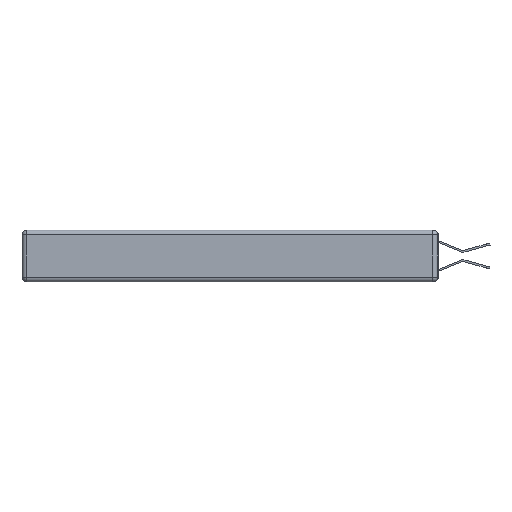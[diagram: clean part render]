
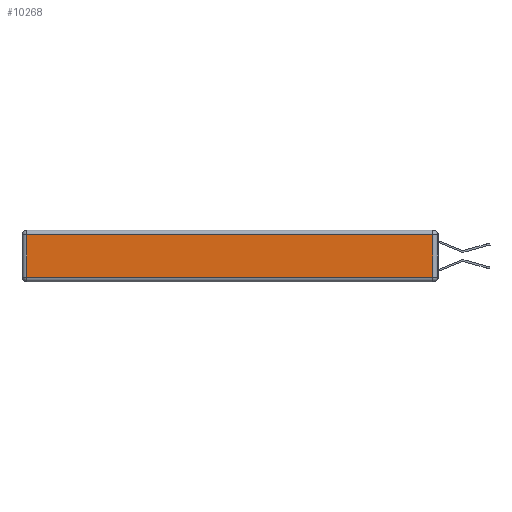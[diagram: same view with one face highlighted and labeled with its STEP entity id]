
A CAD part, left-side view. The second image highlights one B-rep face of the part: STEP entity #10268.
In plain terms, the highlighted planar face has unit normal (-1, 0, 0).
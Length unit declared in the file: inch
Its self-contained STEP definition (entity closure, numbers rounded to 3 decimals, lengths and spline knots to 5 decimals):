
#751 = VERTEX_POINT ( 'NONE', #2397 ) ;
#1025 = VERTEX_POINT ( 'NONE', #12220 ) ;
#1171 = DIRECTION ( 'NONE',  ( 0., 0., 1. ) ) ;
#1710 = CARTESIAN_POINT ( 'NONE',  ( 0., 0.03, -0.313 ) ) ;
#2028 = AXIS2_PLACEMENT_3D ( 'NONE', #13520, #12362, #9829 ) ;
#2120 = CARTESIAN_POINT ( 'NONE',  ( 0., 0., -0.313 ) ) ;
#2397 = CARTESIAN_POINT ( 'NONE',  ( 0., 0.03, -0.03 ) ) ;
#2434 = CARTESIAN_POINT ( 'NONE',  ( 0., 2.72, -0.03 ) ) ;
#2493 = LINE ( 'NONE', #3738, #13508 ) ;
#3329 = FACE_OUTER_BOUND ( 'NONE', #14917, .T. ) ;
#3657 = VECTOR ( 'NONE', #9461, 39.37008 ) ;
#3738 = CARTESIAN_POINT ( 'NONE',  ( 0., 0.03, -0.343 ) ) ;
#4004 = DIRECTION ( 'NONE',  ( 0., 1., 0. ) ) ;
#4325 = LINE ( 'NONE', #15540, #8151 ) ;
#4734 = PLANE ( 'NONE',  #2028 ) ;
#4991 = VECTOR ( 'NONE', #12852, 39.37008 ) ;
#5740 = VERTEX_POINT ( 'NONE', #1710 ) ;
#7200 = LINE ( 'NONE', #2120, #3657 ) ;
#8151 = VECTOR ( 'NONE', #4004, 39.37008 ) ;
#8660 = VERTEX_POINT ( 'NONE', #2434 ) ;
#9112 = EDGE_CURVE ( 'NONE', #5740, #751, #2493, .T. ) ;
#9461 = DIRECTION ( 'NONE',  ( 0., -1., 0. ) ) ;
#9829 = DIRECTION ( 'NONE',  ( 0., 0., 1. ) ) ;
#10151 = EDGE_CURVE ( 'NONE', #751, #8660, #4325, .T. ) ;
#10268 = ADVANCED_FACE ( 'NONE', ( #3329 ), #4734, .T. ) ;
#10754 = ORIENTED_EDGE ( 'NONE', *, *, #11781, .T. ) ;
#11132 = EDGE_CURVE ( 'NONE', #1025, #5740, #7200, .T. ) ;
#11781 = EDGE_CURVE ( 'NONE', #8660, #1025, #13857, .T. ) ;
#12125 = ORIENTED_EDGE ( 'NONE', *, *, #9112, .T. ) ;
#12220 = CARTESIAN_POINT ( 'NONE',  ( 0., 2.72, -0.313 ) ) ;
#12302 = ORIENTED_EDGE ( 'NONE', *, *, #11132, .T. ) ;
#12362 = DIRECTION ( 'NONE',  ( -1., 0., 0. ) ) ;
#12852 = DIRECTION ( 'NONE',  ( 0., 0., -1. ) ) ;
#13508 = VECTOR ( 'NONE', #1171, 39.37008 ) ;
#13520 = CARTESIAN_POINT ( 'NONE',  ( 0., 0., -0.343 ) ) ;
#13857 = LINE ( 'NONE', #15350, #4991 ) ;
#14917 = EDGE_LOOP ( 'NONE', ( #12302, #12125, #15529, #10754 ) ) ;
#15350 = CARTESIAN_POINT ( 'NONE',  ( 0., 2.72, -0.343 ) ) ;
#15529 = ORIENTED_EDGE ( 'NONE', *, *, #10151, .T. ) ;
#15540 = CARTESIAN_POINT ( 'NONE',  ( 0., 2.75, -0.03 ) ) ;
